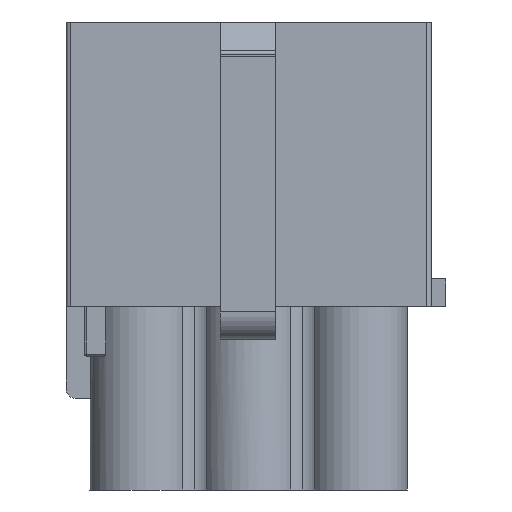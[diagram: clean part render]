
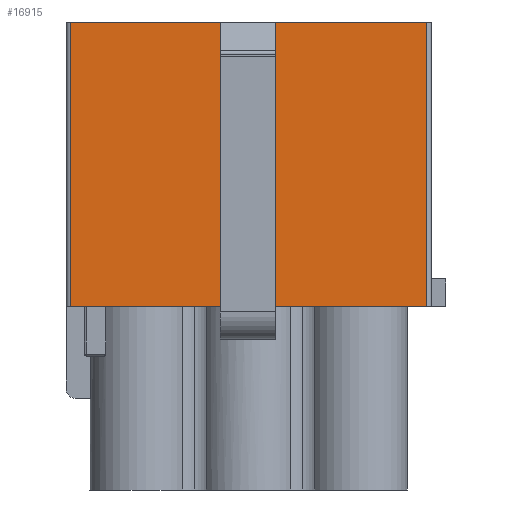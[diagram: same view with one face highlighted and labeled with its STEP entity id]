
A CAD part, left-side view. The second image highlights one B-rep face of the part: STEP entity #16915.
In plain terms, the highlighted planar face has unit normal (-1, 0, 0).
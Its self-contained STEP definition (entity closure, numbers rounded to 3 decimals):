
#304 = VECTOR ( 'NONE', #6679, 1000. ) ;
#530 = VECTOR ( 'NONE', #19753, 1000. ) ;
#815 = VERTEX_POINT ( 'NONE', #8892 ) ;
#1375 = CARTESIAN_POINT ( 'NONE',  ( -8.5, -9.7, -15.5 ) ) ;
#1409 = CARTESIAN_POINT ( 'NONE',  ( -8.5, -1.45, -15.5 ) ) ;
#2131 = DIRECTION ( 'NONE',  ( 0., 1., 0. ) ) ;
#2752 = VECTOR ( 'NONE', #4735, 1000. ) ;
#2971 = VERTEX_POINT ( 'NONE', #14297 ) ;
#3041 = FACE_OUTER_BOUND ( 'NONE', #9071, .T. ) ;
#3167 = DIRECTION ( 'NONE',  ( -1., 0., 0. ) ) ;
#3278 = CARTESIAN_POINT ( 'NONE',  ( -8.5, -9.95, -15.5 ) ) ;
#3283 = ORIENTED_EDGE ( 'NONE', *, *, #15902, .F. ) ;
#4429 = VERTEX_POINT ( 'NONE', #22708 ) ;
#4583 = CARTESIAN_POINT ( 'NONE',  ( -8.5, 1.55, -13.7 ) ) ;
#4735 = DIRECTION ( 'NONE',  ( 0., 0., -1. ) ) ;
#4951 = CARTESIAN_POINT ( 'NONE',  ( -8.5, -9.7, -15.5 ) ) ;
#5084 = ORIENTED_EDGE ( 'NONE', *, *, #10346, .T. ) ;
#6220 = CARTESIAN_POINT ( 'NONE',  ( -8.5, -9.95, 0. ) ) ;
#6224 = VERTEX_POINT ( 'NONE', #14639 ) ;
#6333 = DIRECTION ( 'NONE',  ( 0., -1., 0. ) ) ;
#6435 = VECTOR ( 'NONE', #2131, 1000. ) ;
#6590 = CARTESIAN_POINT ( 'NONE',  ( -8.5, -1.45, -15.5 ) ) ;
#6621 = VERTEX_POINT ( 'NONE', #4583 ) ;
#6679 = DIRECTION ( 'NONE',  ( 0., 0., 1. ) ) ;
#7280 = EDGE_CURVE ( 'NONE', #815, #6621, #10862, .T. ) ;
#8164 = LINE ( 'NONE', #6220, #10074 ) ;
#8242 = VECTOR ( 'NONE', #15660, 1000. ) ;
#8844 = DIRECTION ( 'NONE',  ( 0., 0., -1. ) ) ;
#8892 = CARTESIAN_POINT ( 'NONE',  ( -8.5, -1.45, -13.7 ) ) ;
#9071 = EDGE_LOOP ( 'NONE', ( #5084, #10331, #3283, #18204, #10086, #18144, #13057, #12386 ) ) ;
#9209 = CARTESIAN_POINT ( 'NONE',  ( -8.5, -9.95, -15.5 ) ) ;
#9919 = LINE ( 'NONE', #22214, #2752 ) ;
#10030 = LINE ( 'NONE', #6590, #8242 ) ;
#10074 = VECTOR ( 'NONE', #20109, 1000. ) ;
#10086 = ORIENTED_EDGE ( 'NONE', *, *, #17127, .T. ) ;
#10331 = ORIENTED_EDGE ( 'NONE', *, *, #20073, .T. ) ;
#10346 = EDGE_CURVE ( 'NONE', #11402, #10457, #21604, .T. ) ;
#10457 = VERTEX_POINT ( 'NONE', #1375 ) ;
#10862 = LINE ( 'NONE', #17870, #6435 ) ;
#11402 = VERTEX_POINT ( 'NONE', #1409 ) ;
#12386 = ORIENTED_EDGE ( 'NONE', *, *, #13952, .T. ) ;
#13057 = ORIENTED_EDGE ( 'NONE', *, *, #7280, .F. ) ;
#13952 = EDGE_CURVE ( 'NONE', #815, #11402, #10030, .T. ) ;
#14297 = CARTESIAN_POINT ( 'NONE',  ( -8.5, 1.55, -15.5 ) ) ;
#14639 = CARTESIAN_POINT ( 'NONE',  ( -8.5, -9.7, 0. ) ) ;
#15053 = VECTOR ( 'NONE', #8844, 1000. ) ;
#15140 = CARTESIAN_POINT ( 'NONE',  ( -8.5, 9.7, 0. ) ) ;
#15446 = DIRECTION ( 'NONE',  ( 0., 0., 1. ) ) ;
#15550 = EDGE_CURVE ( 'NONE', #6621, #2971, #9919, .T. ) ;
#15660 = DIRECTION ( 'NONE',  ( 0., 0., -1. ) ) ;
#15902 = EDGE_CURVE ( 'NONE', #17344, #6224, #8164, .T. ) ;
#16727 = AXIS2_PLACEMENT_3D ( 'NONE', #3278, #3167, #15446 ) ;
#16800 = LINE ( 'NONE', #22077, #20022 ) ;
#16915 = ADVANCED_FACE ( 'NONE', ( #3041 ), #20730, .T. ) ;
#17127 = EDGE_CURVE ( 'NONE', #4429, #2971, #16800, .T. ) ;
#17344 = VERTEX_POINT ( 'NONE', #15140 ) ;
#17573 = CARTESIAN_POINT ( 'NONE',  ( -8.5, 9.7, -15.5 ) ) ;
#17870 = CARTESIAN_POINT ( 'NONE',  ( -8.5, -1.45, -13.7 ) ) ;
#18144 = ORIENTED_EDGE ( 'NONE', *, *, #15550, .F. ) ;
#18204 = ORIENTED_EDGE ( 'NONE', *, *, #22723, .T. ) ;
#19753 = DIRECTION ( 'NONE',  ( 0., -1., 0. ) ) ;
#20022 = VECTOR ( 'NONE', #6333, 1000. ) ;
#20073 = EDGE_CURVE ( 'NONE', #10457, #6224, #22421, .T. ) ;
#20109 = DIRECTION ( 'NONE',  ( 0., -1., 0. ) ) ;
#20730 = PLANE ( 'NONE',  #16727 ) ;
#21137 = LINE ( 'NONE', #17573, #15053 ) ;
#21604 = LINE ( 'NONE', #9209, #530 ) ;
#22077 = CARTESIAN_POINT ( 'NONE',  ( -8.5, -9.95, -15.5 ) ) ;
#22214 = CARTESIAN_POINT ( 'NONE',  ( -8.5, 1.55, -15.5 ) ) ;
#22421 = LINE ( 'NONE', #4951, #304 ) ;
#22708 = CARTESIAN_POINT ( 'NONE',  ( -8.5, 9.7, -15.5 ) ) ;
#22723 = EDGE_CURVE ( 'NONE', #17344, #4429, #21137, .T. ) ;
